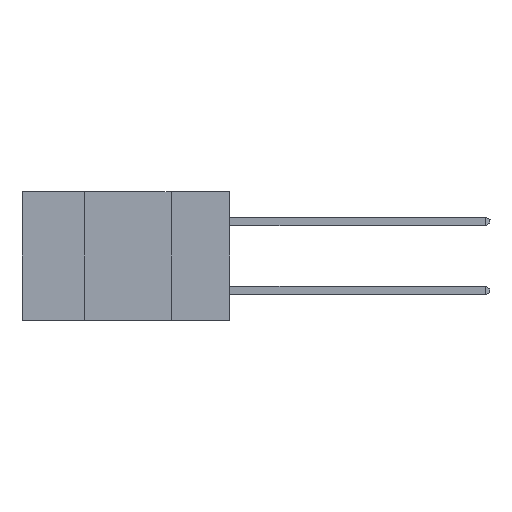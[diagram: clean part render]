
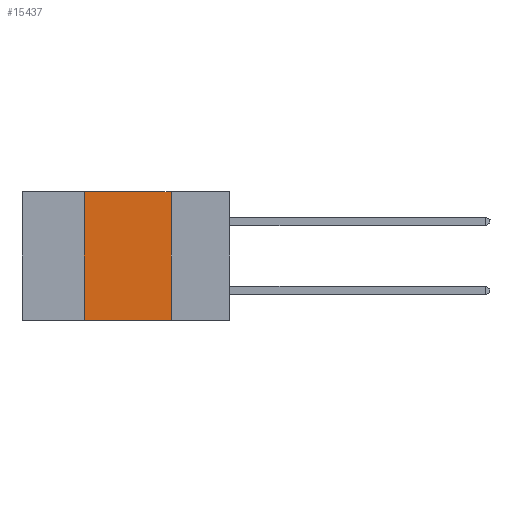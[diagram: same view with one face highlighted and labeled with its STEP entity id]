
A CAD part, left-side view. The second image highlights one B-rep face of the part: STEP entity #15437.
In plain terms, the highlighted planar face has unit normal (-1, 0, 0).
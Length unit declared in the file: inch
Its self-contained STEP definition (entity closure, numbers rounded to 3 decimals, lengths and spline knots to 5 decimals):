
#734 = DIRECTION ( 'NONE',  ( 0., 0., 1. ) ) ;
#749 = CARTESIAN_POINT ( 'NONE',  ( 0., 0.17, 0. ) ) ;
#1283 = LINE ( 'NONE', #21554, #15190 ) ;
#2227 = CARTESIAN_POINT ( 'NONE',  ( 0., 0.6, -0.37 ) ) ;
#3877 = DIRECTION ( 'NONE',  ( 0., -1., 0. ) ) ;
#5168 = ORIENTED_EDGE ( 'NONE', *, *, #6599, .F. ) ;
#5252 = VECTOR ( 'NONE', #15005, 39.37008 ) ;
#5521 = LINE ( 'NONE', #2227, #5252 ) ;
#5685 = CARTESIAN_POINT ( 'NONE',  ( 0., 0.6, 0. ) ) ;
#5959 = PLANE ( 'NONE',  #19002 ) ;
#5963 = VECTOR ( 'NONE', #734, 39.37008 ) ;
#6217 = DIRECTION ( 'NONE',  ( 0., 0., -1. ) ) ;
#6599 = EDGE_CURVE ( 'NONE', #22193, #14472, #6845, .T. ) ;
#6682 = EDGE_LOOP ( 'NONE', ( #18236, #5168, #16315, #6768 ) ) ;
#6768 = ORIENTED_EDGE ( 'NONE', *, *, #18699, .T. ) ;
#6845 = LINE ( 'NONE', #5685, #11063 ) ;
#8587 = VERTEX_POINT ( 'NONE', #14765 ) ;
#9190 = EDGE_CURVE ( 'NONE', #14472, #22841, #1283, .T. ) ;
#9736 = CARTESIAN_POINT ( 'NONE',  ( 0., 0.42, 0. ) ) ;
#10727 = DIRECTION ( 'NONE',  ( 0., 0., -1. ) ) ;
#11063 = VECTOR ( 'NONE', #3877, 39.37008 ) ;
#14472 = VERTEX_POINT ( 'NONE', #749 ) ;
#14765 = CARTESIAN_POINT ( 'NONE',  ( 0., 0.42, -0.37 ) ) ;
#15005 = DIRECTION ( 'NONE',  ( 0., -1., 0. ) ) ;
#15190 = VECTOR ( 'NONE', #10727, 39.37008 ) ;
#15383 = CARTESIAN_POINT ( 'NONE',  ( 0., 0.42, 0. ) ) ;
#15437 = ADVANCED_FACE ( 'NONE', ( #16516 ), #5959, .F. ) ;
#16315 = ORIENTED_EDGE ( 'NONE', *, *, #23061, .F. ) ;
#16516 = FACE_OUTER_BOUND ( 'NONE', #6682, .T. ) ;
#18117 = LINE ( 'NONE', #9736, #5963 ) ;
#18236 = ORIENTED_EDGE ( 'NONE', *, *, #9190, .F. ) ;
#18611 = CARTESIAN_POINT ( 'NONE',  ( 0., 0.6, 0. ) ) ;
#18699 = EDGE_CURVE ( 'NONE', #8587, #22841, #5521, .T. ) ;
#19002 = AXIS2_PLACEMENT_3D ( 'NONE', #18611, #20434, #6217 ) ;
#20434 = DIRECTION ( 'NONE',  ( 1., 0., 0. ) ) ;
#21345 = CARTESIAN_POINT ( 'NONE',  ( 0., 0.17, -0.37 ) ) ;
#21554 = CARTESIAN_POINT ( 'NONE',  ( 0., 0.17, 0. ) ) ;
#22193 = VERTEX_POINT ( 'NONE', #15383 ) ;
#22841 = VERTEX_POINT ( 'NONE', #21345 ) ;
#23061 = EDGE_CURVE ( 'NONE', #8587, #22193, #18117, .T. ) ;
